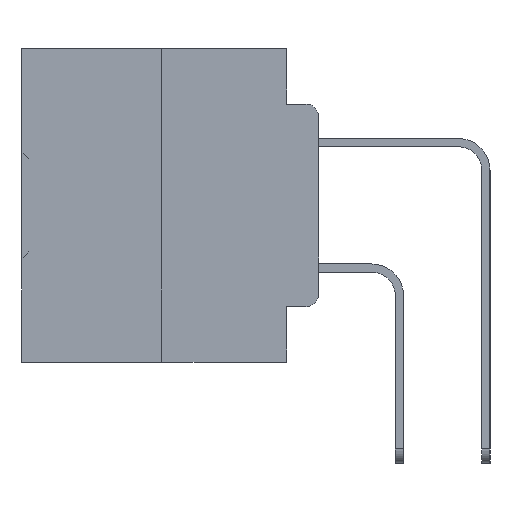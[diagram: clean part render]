
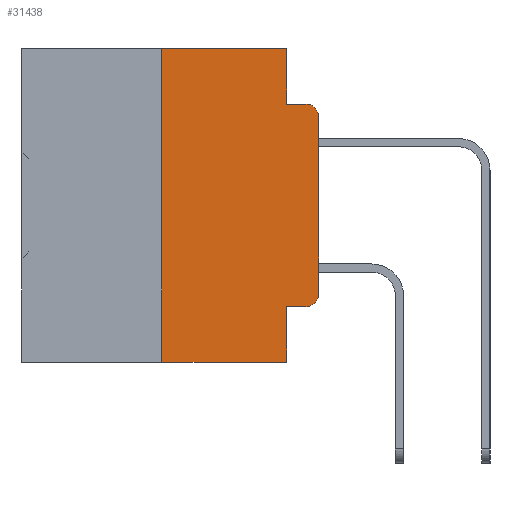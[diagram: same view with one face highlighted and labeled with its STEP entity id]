
A CAD part, left-side view. The second image highlights one B-rep face of the part: STEP entity #31438.
In plain terms, the highlighted planar face has unit normal (-1, 0, 0).
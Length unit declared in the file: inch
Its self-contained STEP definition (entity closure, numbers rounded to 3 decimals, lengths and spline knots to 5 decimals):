
#442 = ORIENTED_EDGE ( 'NONE', *, *, #9667, .T. ) ;
#990 = DIRECTION ( 'NONE',  ( -1., 0., 0. ) ) ;
#1154 = DIRECTION ( 'NONE',  ( 1., 0., 0. ) ) ;
#1552 = ORIENTED_EDGE ( 'NONE', *, *, #13708, .T. ) ;
#1682 = AXIS2_PLACEMENT_3D ( 'NONE', #31707, #14254, #34647 ) ;
#2060 = CARTESIAN_POINT ( 'NONE',  ( 0., 0.051, -0.5 ) ) ;
#2424 = VERTEX_POINT ( 'NONE', #13128 ) ;
#2526 = LINE ( 'NONE', #30557, #9686 ) ;
#2559 = DIRECTION ( 'NONE',  ( 0., -1., 0. ) ) ;
#3367 = DIRECTION ( 'NONE',  ( 0., -1., 0. ) ) ;
#3518 = EDGE_CURVE ( 'NONE', #33562, #2424, #6633, .T. ) ;
#4223 = LINE ( 'NONE', #5182, #20201 ) ;
#5056 = VECTOR ( 'NONE', #2559, 39.37008 ) ;
#5182 = CARTESIAN_POINT ( 'NONE',  ( 0., 0.051, 0. ) ) ;
#6010 = VERTEX_POINT ( 'NONE', #2060 ) ;
#6027 = LINE ( 'NONE', #32100, #5056 ) ;
#6209 = ORIENTED_EDGE ( 'NONE', *, *, #30105, .F. ) ;
#6537 = ORIENTED_EDGE ( 'NONE', *, *, #27904, .T. ) ;
#6633 = LINE ( 'NONE', #33793, #23445 ) ;
#7280 = CIRCLE ( 'NONE', #15684, 0.02 ) ;
#7737 = EDGE_LOOP ( 'NONE', ( #1552, #442, #37232, #37015, #36144, #37690, #6537, #6209, #8557, #8355 ) ) ;
#7905 = CARTESIAN_POINT ( 'NONE',  ( 0., 0., -0.3915 ) ) ;
#8116 = LINE ( 'NONE', #34573, #22056 ) ;
#8206 = DIRECTION ( 'NONE',  ( 0., 0., -1. ) ) ;
#8355 = ORIENTED_EDGE ( 'NONE', *, *, #22311, .T. ) ;
#8488 = VERTEX_POINT ( 'NONE', #27749 ) ;
#8557 = ORIENTED_EDGE ( 'NONE', *, *, #24273, .T. ) ;
#9667 = EDGE_CURVE ( 'NONE', #12648, #2424, #7280, .T. ) ;
#9686 = VECTOR ( 'NONE', #24843, 39.37008 ) ;
#10233 = VECTOR ( 'NONE', #11946, 39.37008 ) ;
#11575 = DIRECTION ( 'NONE',  ( 0., -1., 0. ) ) ;
#11946 = DIRECTION ( 'NONE',  ( 0., 0., 1. ) ) ;
#12034 = CARTESIAN_POINT ( 'NONE',  ( 0., 0.25, 0. ) ) ;
#12459 = CARTESIAN_POINT ( 'NONE',  ( 0., 0.051, -0.0885 ) ) ;
#12589 = VERTEX_POINT ( 'NONE', #37585 ) ;
#12648 = VERTEX_POINT ( 'NONE', #26278 ) ;
#12849 = CIRCLE ( 'NONE', #1682, 0.02 ) ;
#13128 = CARTESIAN_POINT ( 'NONE',  ( 0., 0.02, -0.0885 ) ) ;
#13708 = EDGE_CURVE ( 'NONE', #32241, #12648, #18143, .T. ) ;
#14105 = DIRECTION ( 'NONE',  ( 0., 0., -1. ) ) ;
#14254 = DIRECTION ( 'NONE',  ( -1., 0., 0. ) ) ;
#14895 = VECTOR ( 'NONE', #3367, 39.37008 ) ;
#15684 = AXIS2_PLACEMENT_3D ( 'NONE', #19028, #990, #21984 ) ;
#15689 = FACE_OUTER_BOUND ( 'NONE', #7737, .T. ) ;
#15770 = LINE ( 'NONE', #32757, #14895 ) ;
#17529 = CARTESIAN_POINT ( 'NONE',  ( 0., 0.25, 0. ) ) ;
#18102 = AXIS2_PLACEMENT_3D ( 'NONE', #19190, #1154, #22141 ) ;
#18143 = LINE ( 'NONE', #20737, #10233 ) ;
#19028 = CARTESIAN_POINT ( 'NONE',  ( 0., 0.02, -0.1085 ) ) ;
#19190 = CARTESIAN_POINT ( 'NONE',  ( 0., 0.473, 0. ) ) ;
#20201 = VECTOR ( 'NONE', #14105, 39.37008 ) ;
#20737 = CARTESIAN_POINT ( 'NONE',  ( 0., 0., 0. ) ) ;
#21984 = DIRECTION ( 'NONE',  ( 0., 0., -1. ) ) ;
#22056 = VECTOR ( 'NONE', #8206, 39.37008 ) ;
#22141 = DIRECTION ( 'NONE',  ( 0., 0., -1. ) ) ;
#22311 = EDGE_CURVE ( 'NONE', #35232, #32241, #12849, .T. ) ;
#23445 = VECTOR ( 'NONE', #11575, 39.37008 ) ;
#24273 = EDGE_CURVE ( 'NONE', #8488, #35232, #6027, .T. ) ;
#24843 = DIRECTION ( 'NONE',  ( 0., -1., 0. ) ) ;
#24857 = VERTEX_POINT ( 'NONE', #17529 ) ;
#25421 = CARTESIAN_POINT ( 'NONE',  ( 0., 0.02, -0.4115 ) ) ;
#26278 = CARTESIAN_POINT ( 'NONE',  ( 0., 0., -0.1085 ) ) ;
#26308 = LINE ( 'NONE', #12034, #34017 ) ;
#27625 = VERTEX_POINT ( 'NONE', #31622 ) ;
#27749 = CARTESIAN_POINT ( 'NONE',  ( 0., 0.051, -0.4115 ) ) ;
#27904 = EDGE_CURVE ( 'NONE', #27625, #6010, #2526, .T. ) ;
#30105 = EDGE_CURVE ( 'NONE', #8488, #6010, #4223, .T. ) ;
#30557 = CARTESIAN_POINT ( 'NONE',  ( 0., 0.473, -0.5 ) ) ;
#31438 = ADVANCED_FACE ( 'NONE', ( #15689 ), #36626, .F. ) ;
#31622 = CARTESIAN_POINT ( 'NONE',  ( 0., 0.25, -0.5 ) ) ;
#31707 = CARTESIAN_POINT ( 'NONE',  ( 0., 0.02, -0.3915 ) ) ;
#32100 = CARTESIAN_POINT ( 'NONE',  ( 0., 0.051, -0.4115 ) ) ;
#32241 = VERTEX_POINT ( 'NONE', #7905 ) ;
#32505 = DIRECTION ( 'NONE',  ( 0., 0., 1. ) ) ;
#32757 = CARTESIAN_POINT ( 'NONE',  ( 0., 0.473, 0. ) ) ;
#33562 = VERTEX_POINT ( 'NONE', #12459 ) ;
#33793 = CARTESIAN_POINT ( 'NONE',  ( 0., 0.051, -0.0885 ) ) ;
#34017 = VECTOR ( 'NONE', #32505, 39.37008 ) ;
#34573 = CARTESIAN_POINT ( 'NONE',  ( 0., 0.051, 0. ) ) ;
#34647 = DIRECTION ( 'NONE',  ( 0., 0., -1. ) ) ;
#35232 = VERTEX_POINT ( 'NONE', #25421 ) ;
#35962 = EDGE_CURVE ( 'NONE', #27625, #24857, #26308, .T. ) ;
#36032 = EDGE_CURVE ( 'NONE', #24857, #12589, #15770, .T. ) ;
#36144 = ORIENTED_EDGE ( 'NONE', *, *, #36032, .F. ) ;
#36626 = PLANE ( 'NONE',  #18102 ) ;
#37015 = ORIENTED_EDGE ( 'NONE', *, *, #37911, .F. ) ;
#37232 = ORIENTED_EDGE ( 'NONE', *, *, #3518, .F. ) ;
#37585 = CARTESIAN_POINT ( 'NONE',  ( 0., 0.051, 0. ) ) ;
#37690 = ORIENTED_EDGE ( 'NONE', *, *, #35962, .F. ) ;
#37911 = EDGE_CURVE ( 'NONE', #12589, #33562, #8116, .T. ) ;
